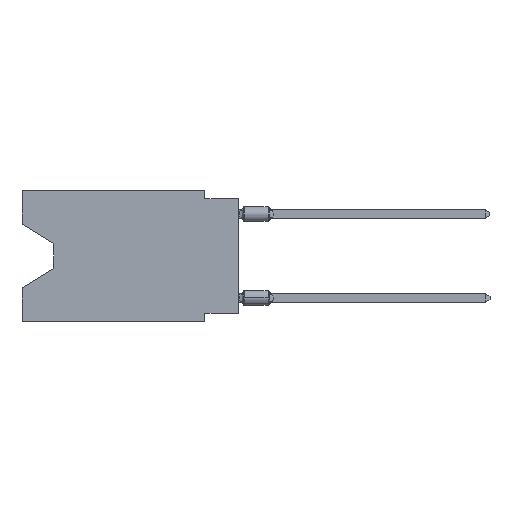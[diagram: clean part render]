
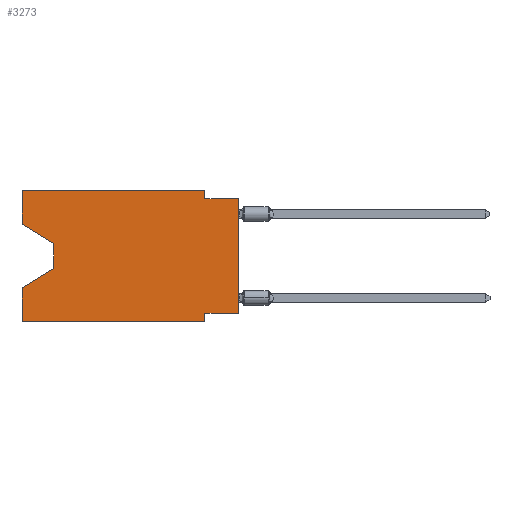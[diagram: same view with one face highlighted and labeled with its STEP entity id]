
A CAD part, left-side view. The second image highlights one B-rep face of the part: STEP entity #3273.
In plain terms, the highlighted planar face has unit normal (-1, 0, 0).
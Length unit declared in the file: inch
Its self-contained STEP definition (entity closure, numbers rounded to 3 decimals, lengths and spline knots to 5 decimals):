
#228 = CARTESIAN_POINT ( 'NONE',  ( 0., 0.645, 0. ) ) ;
#328 = LINE ( 'NONE', #20115, #3768 ) ;
#570 = VECTOR ( 'NONE', #12721, 39.37008 ) ;
#847 = VERTEX_POINT ( 'NONE', #3332 ) ;
#1161 = CARTESIAN_POINT ( 'NONE',  ( 0., 0.645, -0.10025 ) ) ;
#1393 = LINE ( 'NONE', #17181, #7670 ) ;
#1434 = LINE ( 'NONE', #7006, #2426 ) ;
#2058 = LINE ( 'NONE', #228, #22726 ) ;
#2130 = DIRECTION ( 'NONE',  ( 0., 0., 1. ) ) ;
#2426 = VECTOR ( 'NONE', #24743, 39.37008 ) ;
#2560 = CARTESIAN_POINT ( 'NONE',  ( 0., 0.1, -0.365 ) ) ;
#3273 = ADVANCED_FACE ( 'NONE', ( #19020 ), #12825, .F. ) ;
#3282 = EDGE_CURVE ( 'NONE', #847, #8795, #1434, .T. ) ;
#3332 = CARTESIAN_POINT ( 'NONE',  ( 0., 0.645, -0.39 ) ) ;
#3768 = VECTOR ( 'NONE', #16637, 39.37008 ) ;
#3888 = LINE ( 'NONE', #13961, #23323 ) ;
#4747 = EDGE_CURVE ( 'NONE', #22954, #21506, #2058, .T. ) ;
#4829 = CARTESIAN_POINT ( 'NONE',  ( 0., 0.55, -0.232 ) ) ;
#4851 = DIRECTION ( 'NONE',  ( 0., 0., -1. ) ) ;
#4857 = CARTESIAN_POINT ( 'NONE',  ( 0., 0., -0.365 ) ) ;
#4969 = ORIENTED_EDGE ( 'NONE', *, *, #4747, .F. ) ;
#5308 = AXIS2_PLACEMENT_3D ( 'NONE', #10759, #23048, #14771 ) ;
#5350 = EDGE_CURVE ( 'NONE', #14374, #17556, #328, .T. ) ;
#5457 = ORIENTED_EDGE ( 'NONE', *, *, #10993, .F. ) ;
#5918 = ORIENTED_EDGE ( 'NONE', *, *, #8071, .F. ) ;
#7006 = CARTESIAN_POINT ( 'NONE',  ( 0., 0.645, -0.39 ) ) ;
#7399 = VECTOR ( 'NONE', #2130, 39.37008 ) ;
#7670 = VECTOR ( 'NONE', #25082, 39.37008 ) ;
#7927 = EDGE_CURVE ( 'NONE', #21506, #24499, #13007, .T. ) ;
#8062 = LINE ( 'NONE', #15973, #7399 ) ;
#8071 = EDGE_CURVE ( 'NONE', #22244, #13348, #18186, .T. ) ;
#8351 = ORIENTED_EDGE ( 'NONE', *, *, #16748, .T. ) ;
#8584 = CARTESIAN_POINT ( 'NONE',  ( 0., 0.645, 0. ) ) ;
#8795 = VERTEX_POINT ( 'NONE', #14471 ) ;
#9439 = CARTESIAN_POINT ( 'NONE',  ( 0., 0., -0.365 ) ) ;
#9595 = LINE ( 'NONE', #17238, #15236 ) ;
#9712 = EDGE_CURVE ( 'NONE', #15399, #13150, #16612, .T. ) ;
#9864 = CARTESIAN_POINT ( 'NONE',  ( 0., 0.55, -0.232 ) ) ;
#10387 = EDGE_CURVE ( 'NONE', #847, #13150, #3888, .T. ) ;
#10759 = CARTESIAN_POINT ( 'NONE',  ( 0., 0.645, 0. ) ) ;
#10993 = EDGE_CURVE ( 'NONE', #14374, #22954, #14541, .T. ) ;
#11110 = EDGE_LOOP ( 'NONE', ( #22544, #8351, #17178, #18540, #15971, #21417, #5918, #17459, #15040, #23755, #4969, #5457 ) ) ;
#11279 = DIRECTION ( 'NONE',  ( 0., -1., 0. ) ) ;
#11377 = CARTESIAN_POINT ( 'NONE',  ( 0., 0.55, -0.158 ) ) ;
#11675 = VECTOR ( 'NONE', #14431, 39.37008 ) ;
#11986 = EDGE_CURVE ( 'NONE', #13348, #8795, #1393, .T. ) ;
#12721 = DIRECTION ( 'NONE',  ( 0., 0.855, -0.519 ) ) ;
#12744 = CARTESIAN_POINT ( 'NONE',  ( 0., 0.645, 0. ) ) ;
#12825 = PLANE ( 'NONE',  #5308 ) ;
#13007 = LINE ( 'NONE', #19078, #23653 ) ;
#13069 = CARTESIAN_POINT ( 'NONE',  ( 0., 0.645, -0.28975 ) ) ;
#13150 = VERTEX_POINT ( 'NONE', #13069 ) ;
#13183 = CARTESIAN_POINT ( 'NONE',  ( 0., 0., -0.025 ) ) ;
#13348 = VERTEX_POINT ( 'NONE', #2560 ) ;
#13961 = CARTESIAN_POINT ( 'NONE',  ( 0., 0.645, 0. ) ) ;
#14374 = VERTEX_POINT ( 'NONE', #1161 ) ;
#14431 = DIRECTION ( 'NONE',  ( 0., 1., 0. ) ) ;
#14471 = CARTESIAN_POINT ( 'NONE',  ( 0., 0.1, -0.39 ) ) ;
#14541 = LINE ( 'NONE', #8584, #20426 ) ;
#14771 = DIRECTION ( 'NONE',  ( 0., 0., -1. ) ) ;
#15040 = ORIENTED_EDGE ( 'NONE', *, *, #17166, .F. ) ;
#15236 = VECTOR ( 'NONE', #11279, 39.37008 ) ;
#15399 = VERTEX_POINT ( 'NONE', #9864 ) ;
#15971 = ORIENTED_EDGE ( 'NONE', *, *, #3282, .T. ) ;
#15973 = CARTESIAN_POINT ( 'NONE',  ( 0., 0., 0. ) ) ;
#16612 = LINE ( 'NONE', #4829, #570 ) ;
#16634 = LINE ( 'NONE', #24534, #20156 ) ;
#16637 = DIRECTION ( 'NONE',  ( 0., -0.855, -0.519 ) ) ;
#16748 = EDGE_CURVE ( 'NONE', #17556, #15399, #16634, .T. ) ;
#17166 = EDGE_CURVE ( 'NONE', #24499, #20947, #9595, .T. ) ;
#17178 = ORIENTED_EDGE ( 'NONE', *, *, #9712, .T. ) ;
#17181 = CARTESIAN_POINT ( 'NONE',  ( 0., 0.1, -0.39 ) ) ;
#17238 = CARTESIAN_POINT ( 'NONE',  ( 0., 0., -0.025 ) ) ;
#17459 = ORIENTED_EDGE ( 'NONE', *, *, #18048, .T. ) ;
#17556 = VERTEX_POINT ( 'NONE', #11377 ) ;
#17725 = DIRECTION ( 'NONE',  ( 0., 0., 1. ) ) ;
#18048 = EDGE_CURVE ( 'NONE', #22244, #20947, #8062, .T. ) ;
#18186 = LINE ( 'NONE', #4857, #11675 ) ;
#18540 = ORIENTED_EDGE ( 'NONE', *, *, #10387, .F. ) ;
#18953 = DIRECTION ( 'NONE',  ( 0., 0., -1. ) ) ;
#19020 = FACE_OUTER_BOUND ( 'NONE', #11110, .T. ) ;
#19078 = CARTESIAN_POINT ( 'NONE',  ( 0., 0.1, 0. ) ) ;
#20115 = CARTESIAN_POINT ( 'NONE',  ( 0., 0.645, -0.10025 ) ) ;
#20156 = VECTOR ( 'NONE', #4851, 39.37008 ) ;
#20426 = VECTOR ( 'NONE', #23076, 39.37008 ) ;
#20947 = VERTEX_POINT ( 'NONE', #13183 ) ;
#21417 = ORIENTED_EDGE ( 'NONE', *, *, #11986, .F. ) ;
#21506 = VERTEX_POINT ( 'NONE', #24107 ) ;
#21589 = DIRECTION ( 'NONE',  ( 0., -1., 0. ) ) ;
#22244 = VERTEX_POINT ( 'NONE', #9439 ) ;
#22544 = ORIENTED_EDGE ( 'NONE', *, *, #5350, .T. ) ;
#22726 = VECTOR ( 'NONE', #21589, 39.37008 ) ;
#22954 = VERTEX_POINT ( 'NONE', #12744 ) ;
#23048 = DIRECTION ( 'NONE',  ( 1., 0., 0. ) ) ;
#23076 = DIRECTION ( 'NONE',  ( 0., 0., 1. ) ) ;
#23323 = VECTOR ( 'NONE', #17725, 39.37008 ) ;
#23653 = VECTOR ( 'NONE', #18953, 39.37008 ) ;
#23746 = CARTESIAN_POINT ( 'NONE',  ( 0., 0.1, -0.025 ) ) ;
#23755 = ORIENTED_EDGE ( 'NONE', *, *, #7927, .F. ) ;
#24107 = CARTESIAN_POINT ( 'NONE',  ( 0., 0.1, 0. ) ) ;
#24499 = VERTEX_POINT ( 'NONE', #23746 ) ;
#24534 = CARTESIAN_POINT ( 'NONE',  ( 0., 0.55, -0.158 ) ) ;
#24743 = DIRECTION ( 'NONE',  ( 0., -1., 0. ) ) ;
#25082 = DIRECTION ( 'NONE',  ( 0., 0., -1. ) ) ;
